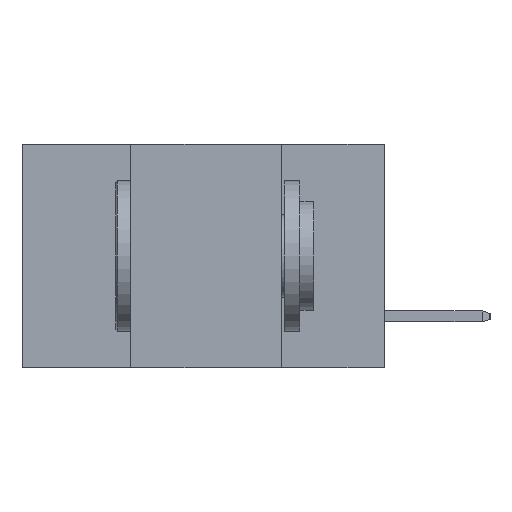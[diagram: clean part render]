
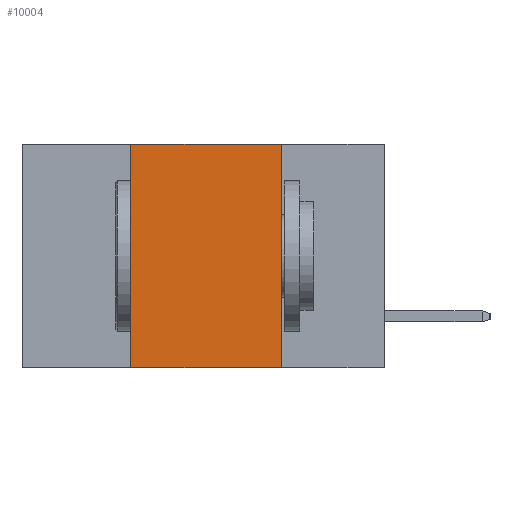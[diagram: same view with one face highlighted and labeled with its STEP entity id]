
A CAD part, left-side view. The second image highlights one B-rep face of the part: STEP entity #10004.
In plain terms, the highlighted planar face has unit normal (-1, 0, 0).
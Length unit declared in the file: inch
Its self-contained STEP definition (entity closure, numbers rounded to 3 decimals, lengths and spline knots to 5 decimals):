
#595 = VECTOR ( 'NONE', #16865, 39.37008 ) ;
#1252 = VECTOR ( 'NONE', #13592, 39.37008 ) ;
#1281 = VERTEX_POINT ( 'NONE', #4169 ) ;
#1553 = LINE ( 'NONE', #9857, #5420 ) ;
#1625 = EDGE_CURVE ( 'NONE', #18174, #15678, #1553, .T. ) ;
#2080 = CARTESIAN_POINT ( 'NONE',  ( 0., 0.42, -0.37 ) ) ;
#2264 = CARTESIAN_POINT ( 'NONE',  ( 0., 0.42, -0.37 ) ) ;
#2600 = VECTOR ( 'NONE', #11936, 39.37008 ) ;
#3393 = CARTESIAN_POINT ( 'NONE',  ( 0., 0.17, -0.37 ) ) ;
#3913 = DIRECTION ( 'NONE',  ( 0., 0., -1. ) ) ;
#3937 = DIRECTION ( 'NONE',  ( 1., 0., 0. ) ) ;
#3954 = PLANE ( 'NONE',  #4643 ) ;
#4004 = LINE ( 'NONE', #7064, #595 ) ;
#4084 = CARTESIAN_POINT ( 'NONE',  ( 0., 0.6, 0. ) ) ;
#4169 = CARTESIAN_POINT ( 'NONE',  ( 0., 0.42, 0. ) ) ;
#4513 = EDGE_LOOP ( 'NONE', ( #13538, #18360, #16041, #7540 ) ) ;
#4643 = AXIS2_PLACEMENT_3D ( 'NONE', #4084, #3937, #3913 ) ;
#5420 = VECTOR ( 'NONE', #10083, 39.37008 ) ;
#5516 = FACE_OUTER_BOUND ( 'NONE', #4513, .T. ) ;
#7064 = CARTESIAN_POINT ( 'NONE',  ( 0., 0.17, -0.37 ) ) ;
#7540 = ORIENTED_EDGE ( 'NONE', *, *, #1625, .T. ) ;
#8517 = LINE ( 'NONE', #2080, #1252 ) ;
#9857 = CARTESIAN_POINT ( 'NONE',  ( 0., 0.6, -0.37 ) ) ;
#10004 = ADVANCED_FACE ( 'NONE', ( #5516 ), #3954, .F. ) ;
#10083 = DIRECTION ( 'NONE',  ( 0., -1., 0. ) ) ;
#11936 = DIRECTION ( 'NONE',  ( 0., -1., 0. ) ) ;
#12996 = VERTEX_POINT ( 'NONE', #13887 ) ;
#13538 = ORIENTED_EDGE ( 'NONE', *, *, #15388, .F. ) ;
#13592 = DIRECTION ( 'NONE',  ( 0., 0., 1. ) ) ;
#13887 = CARTESIAN_POINT ( 'NONE',  ( 0., 0.17, 0. ) ) ;
#14044 = LINE ( 'NONE', #14691, #2600 ) ;
#14691 = CARTESIAN_POINT ( 'NONE',  ( 0., 0.6, 0. ) ) ;
#15388 = EDGE_CURVE ( 'NONE', #12996, #15678, #4004, .T. ) ;
#15678 = VERTEX_POINT ( 'NONE', #3393 ) ;
#16041 = ORIENTED_EDGE ( 'NONE', *, *, #18077, .F. ) ;
#16273 = EDGE_CURVE ( 'NONE', #1281, #12996, #14044, .T. ) ;
#16865 = DIRECTION ( 'NONE',  ( 0., 0., -1. ) ) ;
#18077 = EDGE_CURVE ( 'NONE', #18174, #1281, #8517, .T. ) ;
#18174 = VERTEX_POINT ( 'NONE', #2264 ) ;
#18360 = ORIENTED_EDGE ( 'NONE', *, *, #16273, .F. ) ;
